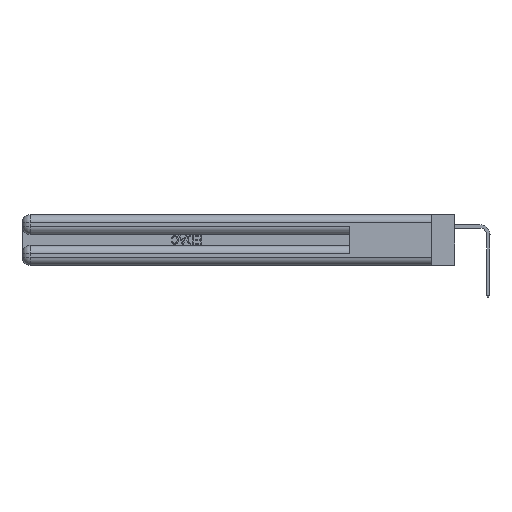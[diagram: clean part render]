
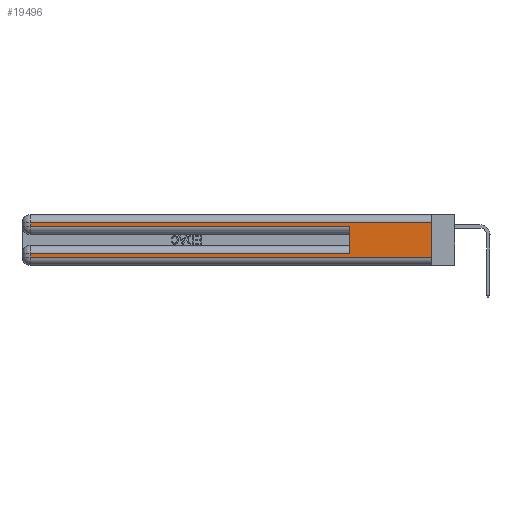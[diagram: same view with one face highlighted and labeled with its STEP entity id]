
A CAD part, left-side view. The second image highlights one B-rep face of the part: STEP entity #19496.
In plain terms, the highlighted planar face has unit normal (-1, 0, 0).
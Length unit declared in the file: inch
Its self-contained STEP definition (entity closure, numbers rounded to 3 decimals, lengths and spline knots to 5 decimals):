
#59 = VERTEX_POINT ( 'NONE', #27029 ) ;
#1405 = VERTEX_POINT ( 'NONE', #30841 ) ;
#1989 = ORIENTED_EDGE ( 'NONE', *, *, #38998, .T. ) ;
#2534 = VECTOR ( 'NONE', #17046, 39.37008 ) ;
#4960 = EDGE_CURVE ( 'NONE', #34141, #5232, #13910, .T. ) ;
#5007 = EDGE_CURVE ( 'NONE', #27776, #20450, #33084, .T. ) ;
#5232 = VERTEX_POINT ( 'NONE', #32912 ) ;
#6062 = VERTEX_POINT ( 'NONE', #45895 ) ;
#6768 = LINE ( 'NONE', #37406, #46481 ) ;
#8342 = LINE ( 'NONE', #8787, #30110 ) ;
#8787 = CARTESIAN_POINT ( 'NONE',  ( 0., 2.94, 0.37 ) ) ;
#9274 = LINE ( 'NONE', #13532, #51584 ) ;
#11624 = ORIENTED_EDGE ( 'NONE', *, *, #23525, .T. ) ;
#12286 = EDGE_CURVE ( 'NONE', #6062, #34141, #13458, .T. ) ;
#12651 = VECTOR ( 'NONE', #14852, 39.37008 ) ;
#12915 = DIRECTION ( 'NONE',  ( 0., 0., -1. ) ) ;
#13076 = CARTESIAN_POINT ( 'NONE',  ( 0., 0., 0.31 ) ) ;
#13458 = LINE ( 'NONE', #45690, #2534 ) ;
#13532 = CARTESIAN_POINT ( 'NONE',  ( 0., 0., 0.37 ) ) ;
#13910 = LINE ( 'NONE', #39397, #45252 ) ;
#14852 = DIRECTION ( 'NONE',  ( 0., 0., 1. ) ) ;
#17046 = DIRECTION ( 'NONE',  ( 0., 1., 0. ) ) ;
#18644 = ORIENTED_EDGE ( 'NONE', *, *, #52003, .F. ) ;
#18666 = DIRECTION ( 'NONE',  ( 0., -1., 0. ) ) ;
#19013 = EDGE_CURVE ( 'NONE', #5232, #59, #46975, .T. ) ;
#19483 = AXIS2_PLACEMENT_3D ( 'NONE', #42072, #21663, #50327 ) ;
#19496 = ADVANCED_FACE ( 'NONE', ( #33478 ), #41894, .F. ) ;
#19978 = ORIENTED_EDGE ( 'NONE', *, *, #4960, .T. ) ;
#20450 = VERTEX_POINT ( 'NONE', #52919 ) ;
#21663 = DIRECTION ( 'NONE',  ( 1., 0., 0. ) ) ;
#22180 = VECTOR ( 'NONE', #35453, 39.37008 ) ;
#22893 = CARTESIAN_POINT ( 'NONE',  ( 0., 0.6, 0.145 ) ) ;
#23525 = EDGE_CURVE ( 'NONE', #37376, #1405, #6768, .T. ) ;
#23914 = VECTOR ( 'NONE', #18666, 39.37008 ) ;
#27029 = CARTESIAN_POINT ( 'NONE',  ( 0., 0., 0.06 ) ) ;
#27776 = VERTEX_POINT ( 'NONE', #31908 ) ;
#30110 = VECTOR ( 'NONE', #12915, 39.37008 ) ;
#30841 = CARTESIAN_POINT ( 'NONE',  ( 0., 2.94, 0.31 ) ) ;
#31327 = CARTESIAN_POINT ( 'NONE',  ( 0., 0., 0.285 ) ) ;
#31908 = CARTESIAN_POINT ( 'NONE',  ( 0., 2.94, 0.285 ) ) ;
#32912 = CARTESIAN_POINT ( 'NONE',  ( 0., 2.94, 0.06 ) ) ;
#33084 = LINE ( 'NONE', #31327, #22180 ) ;
#33478 = FACE_OUTER_BOUND ( 'NONE', #37874, .T. ) ;
#34141 = VERTEX_POINT ( 'NONE', #42755 ) ;
#34249 = EDGE_CURVE ( 'NONE', #6062, #20450, #45306, .T. ) ;
#35453 = DIRECTION ( 'NONE',  ( 0., -1., 0. ) ) ;
#37260 = ORIENTED_EDGE ( 'NONE', *, *, #5007, .T. ) ;
#37376 = VERTEX_POINT ( 'NONE', #13076 ) ;
#37406 = CARTESIAN_POINT ( 'NONE',  ( 0., 0., 0.31 ) ) ;
#37874 = EDGE_LOOP ( 'NONE', ( #18644, #11624, #1989, #37260, #49441, #37926, #19978, #52660 ) ) ;
#37926 = ORIENTED_EDGE ( 'NONE', *, *, #12286, .T. ) ;
#38998 = EDGE_CURVE ( 'NONE', #1405, #27776, #8342, .T. ) ;
#39102 = CARTESIAN_POINT ( 'NONE',  ( 0., 0., 0.06 ) ) ;
#39397 = CARTESIAN_POINT ( 'NONE',  ( 0., 2.94, 0.37 ) ) ;
#41517 = DIRECTION ( 'NONE',  ( 0., 1., 0. ) ) ;
#41894 = PLANE ( 'NONE',  #19483 ) ;
#42072 = CARTESIAN_POINT ( 'NONE',  ( 0., 0., 0.37 ) ) ;
#42755 = CARTESIAN_POINT ( 'NONE',  ( 0., 2.94, 0.085 ) ) ;
#43497 = DIRECTION ( 'NONE',  ( 0., 0., -1. ) ) ;
#45252 = VECTOR ( 'NONE', #43497, 39.37008 ) ;
#45306 = LINE ( 'NONE', #22893, #12651 ) ;
#45690 = CARTESIAN_POINT ( 'NONE',  ( 0., 0., 0.085 ) ) ;
#45895 = CARTESIAN_POINT ( 'NONE',  ( 0., 0.6, 0.085 ) ) ;
#46481 = VECTOR ( 'NONE', #41517, 39.37008 ) ;
#46975 = LINE ( 'NONE', #39102, #23914 ) ;
#49441 = ORIENTED_EDGE ( 'NONE', *, *, #34249, .F. ) ;
#50327 = DIRECTION ( 'NONE',  ( 0., 0., -1. ) ) ;
#50406 = DIRECTION ( 'NONE',  ( 0., 0., -1. ) ) ;
#51584 = VECTOR ( 'NONE', #50406, 39.37008 ) ;
#52003 = EDGE_CURVE ( 'NONE', #37376, #59, #9274, .T. ) ;
#52660 = ORIENTED_EDGE ( 'NONE', *, *, #19013, .T. ) ;
#52919 = CARTESIAN_POINT ( 'NONE',  ( 0., 0.6, 0.285 ) ) ;
